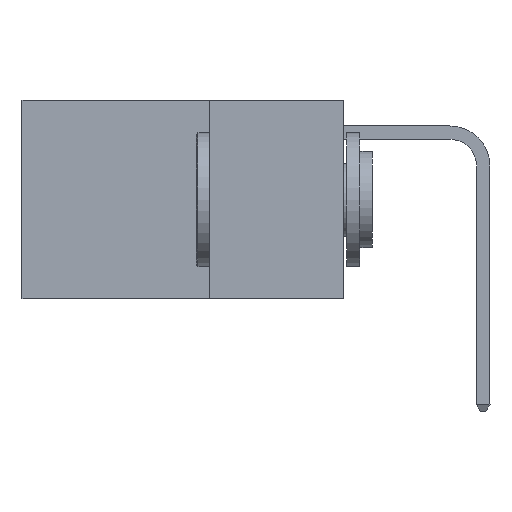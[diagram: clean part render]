
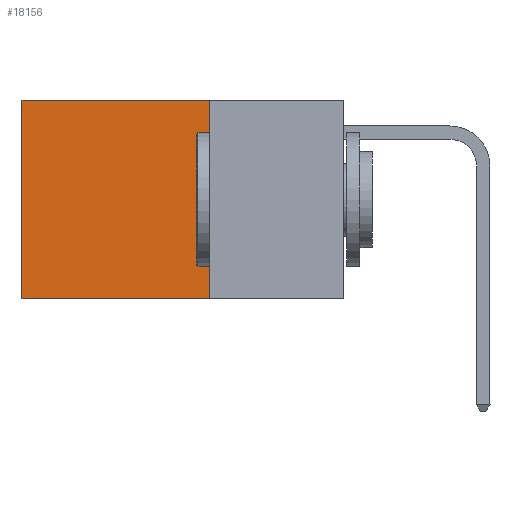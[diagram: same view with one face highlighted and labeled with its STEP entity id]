
A CAD part, left-side view. The second image highlights one B-rep face of the part: STEP entity #18156.
In plain terms, the highlighted planar face has unit normal (-1, 0, 0).
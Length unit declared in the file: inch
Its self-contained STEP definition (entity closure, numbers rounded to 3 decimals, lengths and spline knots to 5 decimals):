
#252 = FACE_OUTER_BOUND ( 'NONE', #5070, .T. ) ;
#392 = VERTEX_POINT ( 'NONE', #19905 ) ;
#620 = VERTEX_POINT ( 'NONE', #9065 ) ;
#1543 = PLANE ( 'NONE',  #11250 ) ;
#2407 = CARTESIAN_POINT ( 'NONE',  ( 0.2625, 0.25, 0. ) ) ;
#4624 = ORIENTED_EDGE ( 'NONE', *, *, #18805, .F. ) ;
#4660 = DIRECTION ( 'NONE',  ( 1., 0., 0. ) ) ;
#5070 = EDGE_LOOP ( 'NONE', ( #10599, #4624, #12593, #14081 ) ) ;
#5345 = CARTESIAN_POINT ( 'NONE',  ( 0.2625, 0.25, -0.37 ) ) ;
#5445 = EDGE_CURVE ( 'NONE', #10441, #392, #7253, .T. ) ;
#6524 = LINE ( 'NONE', #13798, #18868 ) ;
#7253 = LINE ( 'NONE', #9120, #19109 ) ;
#9037 = DIRECTION ( 'NONE',  ( 0., 0., -1. ) ) ;
#9065 = CARTESIAN_POINT ( 'NONE',  ( 0.2625, 0.25, 0. ) ) ;
#9120 = CARTESIAN_POINT ( 'NONE',  ( 0.2625, 0.6, 0. ) ) ;
#9196 = DIRECTION ( 'NONE',  ( 0., 0., -1. ) ) ;
#10441 = VERTEX_POINT ( 'NONE', #18945 ) ;
#10568 = VECTOR ( 'NONE', #11691, 39.37008 ) ;
#10599 = ORIENTED_EDGE ( 'NONE', *, *, #5445, .T. ) ;
#11031 = LINE ( 'NONE', #2407, #10568 ) ;
#11250 = AXIS2_PLACEMENT_3D ( 'NONE', #13937, #4660, #15484 ) ;
#11691 = DIRECTION ( 'NONE',  ( 0., 1., 0. ) ) ;
#11814 = VERTEX_POINT ( 'NONE', #16860 ) ;
#12593 = ORIENTED_EDGE ( 'NONE', *, *, #16215, .F. ) ;
#12600 = EDGE_CURVE ( 'NONE', #620, #10441, #11031, .T. ) ;
#12832 = VECTOR ( 'NONE', #19255, 39.37008 ) ;
#13798 = CARTESIAN_POINT ( 'NONE',  ( 0.2625, 0.25, 0. ) ) ;
#13937 = CARTESIAN_POINT ( 'NONE',  ( 0.2625, 0.25, 0. ) ) ;
#14081 = ORIENTED_EDGE ( 'NONE', *, *, #12600, .T. ) ;
#15484 = DIRECTION ( 'NONE',  ( 0., 0., -1. ) ) ;
#16215 = EDGE_CURVE ( 'NONE', #620, #11814, #6524, .T. ) ;
#16860 = CARTESIAN_POINT ( 'NONE',  ( 0.2625, 0.25, -0.37 ) ) ;
#17405 = LINE ( 'NONE', #5345, #12832 ) ;
#18156 = ADVANCED_FACE ( 'NONE', ( #252 ), #1543, .F. ) ;
#18805 = EDGE_CURVE ( 'NONE', #11814, #392, #17405, .T. ) ;
#18868 = VECTOR ( 'NONE', #9196, 39.37008 ) ;
#18945 = CARTESIAN_POINT ( 'NONE',  ( 0.2625, 0.6, 0. ) ) ;
#19109 = VECTOR ( 'NONE', #9037, 39.37008 ) ;
#19255 = DIRECTION ( 'NONE',  ( 0., 1., 0. ) ) ;
#19905 = CARTESIAN_POINT ( 'NONE',  ( 0.2625, 0.6, -0.37 ) ) ;
